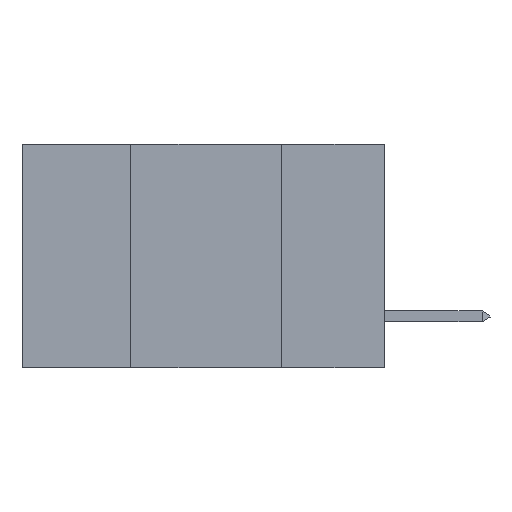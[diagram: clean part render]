
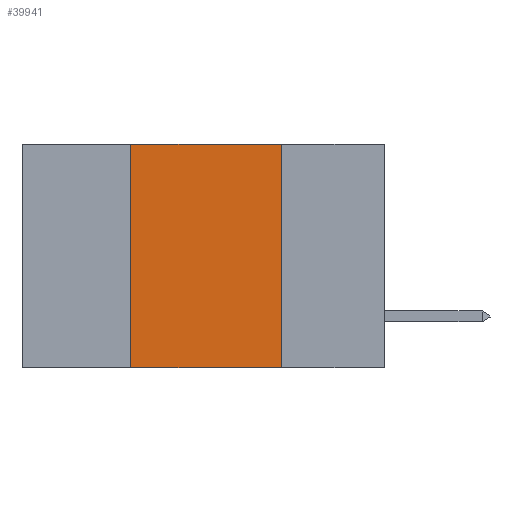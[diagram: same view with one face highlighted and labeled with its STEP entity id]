
A CAD part, left-side view. The second image highlights one B-rep face of the part: STEP entity #39941.
In plain terms, the highlighted planar face has unit normal (-1, 0, 0).
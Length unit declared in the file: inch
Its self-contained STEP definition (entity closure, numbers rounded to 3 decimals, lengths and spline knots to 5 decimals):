
#254 = VERTEX_POINT ( 'NONE', #15638 ) ;
#572 = PLANE ( 'NONE',  #1906 ) ;
#1350 = LINE ( 'NONE', #35990, #9353 ) ;
#1826 = VERTEX_POINT ( 'NONE', #39616 ) ;
#1906 = AXIS2_PLACEMENT_3D ( 'NONE', #35414, #19560, #22760 ) ;
#3028 = ORIENTED_EDGE ( 'NONE', *, *, #40927, .T. ) ;
#3746 = CARTESIAN_POINT ( 'NONE',  ( 0., 0.17, 0. ) ) ;
#3774 = CARTESIAN_POINT ( 'NONE',  ( 0., 0.17, 0. ) ) ;
#4023 = DIRECTION ( 'NONE',  ( 0., 0., -1. ) ) ;
#5293 = ORIENTED_EDGE ( 'NONE', *, *, #28571, .F. ) ;
#8598 = VERTEX_POINT ( 'NONE', #28947 ) ;
#8955 = CARTESIAN_POINT ( 'NONE',  ( 0., 0.6, -0.37 ) ) ;
#9353 = VECTOR ( 'NONE', #29599, 39.37008 ) ;
#10402 = ORIENTED_EDGE ( 'NONE', *, *, #17097, .F. ) ;
#15638 = CARTESIAN_POINT ( 'NONE',  ( 0., 0.42, -0.37 ) ) ;
#15955 = DIRECTION ( 'NONE',  ( 0., 0., 1. ) ) ;
#16771 = LINE ( 'NONE', #8955, #30157 ) ;
#17097 = EDGE_CURVE ( 'NONE', #34196, #8598, #23123, .T. ) ;
#19560 = DIRECTION ( 'NONE',  ( 1., 0., 0. ) ) ;
#22753 = LINE ( 'NONE', #38002, #40659 ) ;
#22760 = DIRECTION ( 'NONE',  ( 0., 0., -1. ) ) ;
#23123 = LINE ( 'NONE', #3746, #26578 ) ;
#24912 = DIRECTION ( 'NONE',  ( 0., -1., 0. ) ) ;
#26578 = VECTOR ( 'NONE', #4023, 39.37008 ) ;
#27195 = EDGE_LOOP ( 'NONE', ( #10402, #5293, #39848, #3028 ) ) ;
#28571 = EDGE_CURVE ( 'NONE', #1826, #34196, #1350, .T. ) ;
#28947 = CARTESIAN_POINT ( 'NONE',  ( 0., 0.17, -0.37 ) ) ;
#29599 = DIRECTION ( 'NONE',  ( 0., -1., 0. ) ) ;
#30157 = VECTOR ( 'NONE', #24912, 39.37008 ) ;
#32777 = FACE_OUTER_BOUND ( 'NONE', #27195, .T. ) ;
#34196 = VERTEX_POINT ( 'NONE', #3774 ) ;
#35414 = CARTESIAN_POINT ( 'NONE',  ( 0., 0.6, 0. ) ) ;
#35990 = CARTESIAN_POINT ( 'NONE',  ( 0., 0.6, 0. ) ) ;
#38002 = CARTESIAN_POINT ( 'NONE',  ( 0., 0.42, 0. ) ) ;
#39616 = CARTESIAN_POINT ( 'NONE',  ( 0., 0.42, 0. ) ) ;
#39848 = ORIENTED_EDGE ( 'NONE', *, *, #40393, .F. ) ;
#39941 = ADVANCED_FACE ( 'NONE', ( #32777 ), #572, .F. ) ;
#40393 = EDGE_CURVE ( 'NONE', #254, #1826, #22753, .T. ) ;
#40659 = VECTOR ( 'NONE', #15955, 39.37008 ) ;
#40927 = EDGE_CURVE ( 'NONE', #254, #8598, #16771, .T. ) ;
